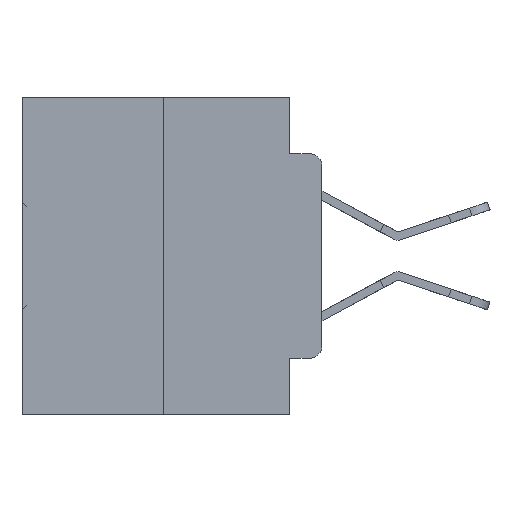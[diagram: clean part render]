
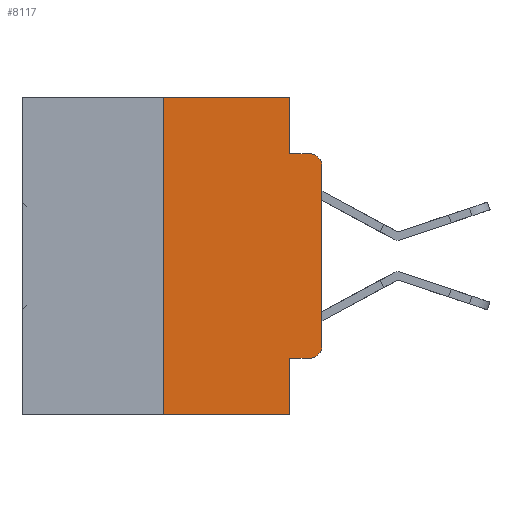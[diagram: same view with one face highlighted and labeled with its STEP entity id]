
A CAD part, left-side view. The second image highlights one B-rep face of the part: STEP entity #8117.
In plain terms, the highlighted planar face has unit normal (-1, 0, 0).
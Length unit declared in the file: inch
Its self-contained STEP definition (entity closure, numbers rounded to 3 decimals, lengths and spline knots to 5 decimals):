
#159 = EDGE_CURVE ( 'NONE', #7119, #3471, #12696, .T. ) ;
#373 = ORIENTED_EDGE ( 'NONE', *, *, #26467, .T. ) ;
#702 = VERTEX_POINT ( 'NONE', #24626 ) ;
#1232 = EDGE_LOOP ( 'NONE', ( #373, #29593, #6419, #23709, #4992, #3911, #23438, #15019, #4906, #33784 ) ) ;
#1285 = DIRECTION ( 'NONE',  ( 0., -1., 0. ) ) ;
#1768 = DIRECTION ( 'NONE',  ( 0., 0., -1. ) ) ;
#1987 = DIRECTION ( 'NONE',  ( 0., -1., 0. ) ) ;
#2279 = LINE ( 'NONE', #19620, #22929 ) ;
#2458 = CARTESIAN_POINT ( 'NONE',  ( 0., 0.051, -0.4115 ) ) ;
#2791 = EDGE_CURVE ( 'NONE', #28643, #33863, #2279, .T. ) ;
#3159 = DIRECTION ( 'NONE',  ( 0., 0., -1. ) ) ;
#3471 = VERTEX_POINT ( 'NONE', #3922 ) ;
#3808 = AXIS2_PLACEMENT_3D ( 'NONE', #28107, #12111, #30766 ) ;
#3911 = ORIENTED_EDGE ( 'NONE', *, *, #32023, .F. ) ;
#3922 = CARTESIAN_POINT ( 'NONE',  ( 0., 0.02, -0.0885 ) ) ;
#3952 = VERTEX_POINT ( 'NONE', #11404 ) ;
#4278 = CARTESIAN_POINT ( 'NONE',  ( 0., 0., -0.3915 ) ) ;
#4906 = ORIENTED_EDGE ( 'NONE', *, *, #2791, .T. ) ;
#4992 = ORIENTED_EDGE ( 'NONE', *, *, #16067, .F. ) ;
#6003 = VERTEX_POINT ( 'NONE', #25146 ) ;
#6419 = ORIENTED_EDGE ( 'NONE', *, *, #12007, .F. ) ;
#6926 = AXIS2_PLACEMENT_3D ( 'NONE', #33925, #17996, #1768 ) ;
#7119 = VERTEX_POINT ( 'NONE', #34667 ) ;
#8117 = ADVANCED_FACE ( 'NONE', ( #32006 ), #25904, .F. ) ;
#8387 = VECTOR ( 'NONE', #10342, 39.37008 ) ;
#8740 = EDGE_CURVE ( 'NONE', #28643, #6003, #26986, .T. ) ;
#8746 = VERTEX_POINT ( 'NONE', #4278 ) ;
#8983 = VECTOR ( 'NONE', #9986, 39.37008 ) ;
#9866 = DIRECTION ( 'NONE',  ( 0., 0., -1. ) ) ;
#9986 = DIRECTION ( 'NONE',  ( 0., -1., 0. ) ) ;
#10342 = DIRECTION ( 'NONE',  ( 0., 0., 1. ) ) ;
#11404 = CARTESIAN_POINT ( 'NONE',  ( 0., 0.051, 0. ) ) ;
#11988 = EDGE_CURVE ( 'NONE', #32612, #6003, #16153, .T. ) ;
#12007 = EDGE_CURVE ( 'NONE', #702, #3471, #22362, .T. ) ;
#12111 = DIRECTION ( 'NONE',  ( -1., 0., 0. ) ) ;
#12696 = CIRCLE ( 'NONE', #21356, 0.02 ) ;
#12705 = CARTESIAN_POINT ( 'NONE',  ( 0., 0.473, -0.5 ) ) ;
#13852 = VERTEX_POINT ( 'NONE', #32673 ) ;
#14640 = VECTOR ( 'NONE', #1285, 39.37008 ) ;
#15019 = ORIENTED_EDGE ( 'NONE', *, *, #8740, .F. ) ;
#15311 = VECTOR ( 'NONE', #1987, 39.37008 ) ;
#16067 = EDGE_CURVE ( 'NONE', #13852, #3952, #21705, .T. ) ;
#16153 = LINE ( 'NONE', #12705, #8983 ) ;
#16853 = DIRECTION ( 'NONE',  ( 0., 0., 1. ) ) ;
#17996 = DIRECTION ( 'NONE',  ( 1., 0., 0. ) ) ;
#19165 = CARTESIAN_POINT ( 'NONE',  ( 0., 0.02, -0.4115 ) ) ;
#19613 = LINE ( 'NONE', #30104, #24177 ) ;
#19620 = CARTESIAN_POINT ( 'NONE',  ( 0., 0.051, -0.4115 ) ) ;
#20359 = CIRCLE ( 'NONE', #3808, 0.02 ) ;
#21356 = AXIS2_PLACEMENT_3D ( 'NONE', #27132, #29184, #29178 ) ;
#21705 = LINE ( 'NONE', #22767, #14640 ) ;
#21979 = CARTESIAN_POINT ( 'NONE',  ( 0., 0.051, 0. ) ) ;
#22362 = LINE ( 'NONE', #28789, #15311 ) ;
#22767 = CARTESIAN_POINT ( 'NONE',  ( 0., 0.473, 0. ) ) ;
#22929 = VECTOR ( 'NONE', #24959, 39.37008 ) ;
#23438 = ORIENTED_EDGE ( 'NONE', *, *, #11988, .T. ) ;
#23709 = ORIENTED_EDGE ( 'NONE', *, *, #31366, .F. ) ;
#24177 = VECTOR ( 'NONE', #16853, 39.37008 ) ;
#24626 = CARTESIAN_POINT ( 'NONE',  ( 0., 0.051, -0.0885 ) ) ;
#24959 = DIRECTION ( 'NONE',  ( 0., -1., 0. ) ) ;
#25055 = CARTESIAN_POINT ( 'NONE',  ( 0., 0.25, -0.5 ) ) ;
#25146 = CARTESIAN_POINT ( 'NONE',  ( 0., 0.051, -0.5 ) ) ;
#25864 = CARTESIAN_POINT ( 'NONE',  ( 0., 0.051, 0. ) ) ;
#25904 = PLANE ( 'NONE',  #6926 ) ;
#26467 = EDGE_CURVE ( 'NONE', #8746, #7119, #28074, .T. ) ;
#26986 = LINE ( 'NONE', #25864, #34034 ) ;
#27132 = CARTESIAN_POINT ( 'NONE',  ( 0., 0.02, -0.1085 ) ) ;
#28074 = LINE ( 'NONE', #29027, #8387 ) ;
#28107 = CARTESIAN_POINT ( 'NONE',  ( 0., 0.02, -0.3915 ) ) ;
#28643 = VERTEX_POINT ( 'NONE', #2458 ) ;
#28789 = CARTESIAN_POINT ( 'NONE',  ( 0., 0.051, -0.0885 ) ) ;
#29027 = CARTESIAN_POINT ( 'NONE',  ( 0., 0., 0. ) ) ;
#29178 = DIRECTION ( 'NONE',  ( 0., 0., -1. ) ) ;
#29184 = DIRECTION ( 'NONE',  ( -1., 0., 0. ) ) ;
#29593 = ORIENTED_EDGE ( 'NONE', *, *, #159, .T. ) ;
#30064 = VECTOR ( 'NONE', #3159, 39.37008 ) ;
#30104 = CARTESIAN_POINT ( 'NONE',  ( 0., 0.25, 0. ) ) ;
#30766 = DIRECTION ( 'NONE',  ( 0., 0., -1. ) ) ;
#30900 = LINE ( 'NONE', #21979, #30064 ) ;
#31366 = EDGE_CURVE ( 'NONE', #3952, #702, #30900, .T. ) ;
#32006 = FACE_OUTER_BOUND ( 'NONE', #1232, .T. ) ;
#32023 = EDGE_CURVE ( 'NONE', #32612, #13852, #19613, .T. ) ;
#32612 = VERTEX_POINT ( 'NONE', #25055 ) ;
#32673 = CARTESIAN_POINT ( 'NONE',  ( 0., 0.25, 0. ) ) ;
#32683 = EDGE_CURVE ( 'NONE', #33863, #8746, #20359, .T. ) ;
#33784 = ORIENTED_EDGE ( 'NONE', *, *, #32683, .T. ) ;
#33863 = VERTEX_POINT ( 'NONE', #19165 ) ;
#33925 = CARTESIAN_POINT ( 'NONE',  ( 0., 0.473, 0. ) ) ;
#34034 = VECTOR ( 'NONE', #9866, 39.37008 ) ;
#34667 = CARTESIAN_POINT ( 'NONE',  ( 0., 0., -0.1085 ) ) ;
